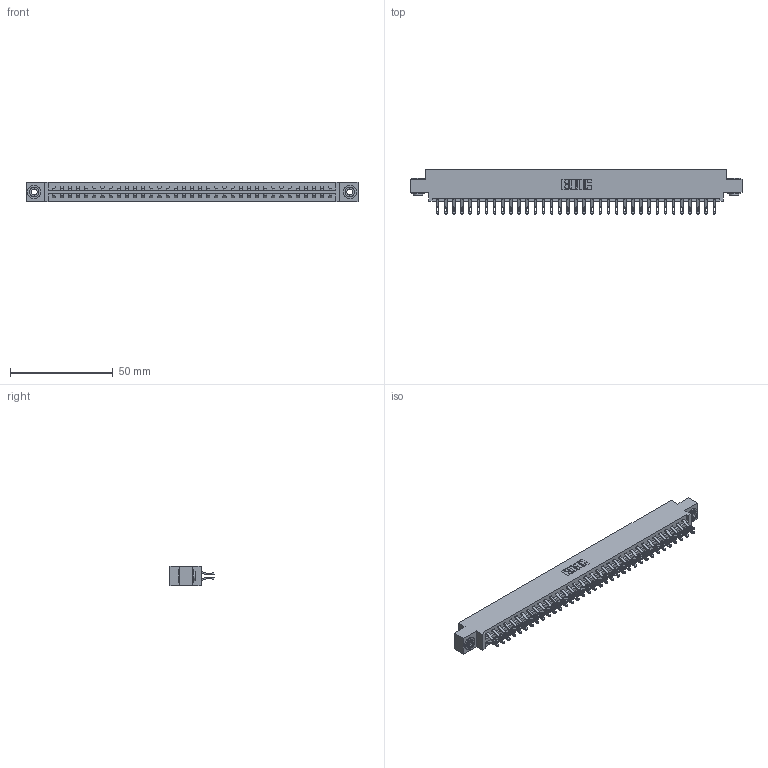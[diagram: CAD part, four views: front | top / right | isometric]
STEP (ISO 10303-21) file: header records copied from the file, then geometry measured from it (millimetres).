
FILE_DESCRIPTION (( 'STEP AP203' ), '1' );
FILE_NAME ('387-070-555-803.STEP', '2018-09-22T17:11:37', ( '' ), ( '' ), 'SwSTEP 2.0', 'SolidWorks 2016', '' );
FILE_SCHEMA (( 'CONFIG_CONTROL_DESIGN' ));
Length unit declared in the file: inch
Products named in the file (4): 337 Part_0.170 Offset - 0.156 Dia-TH; 345-292-001_555 Tail; 345-250-002_345-250-002-102; 387-070-555-803
Assembly tree (73 placements, depth 2):
  387-070-555-803
    337 Part_0.170 Offset - 0.156 Dia-TH
    345-292-001_555 Tail  x70
    345-250-002_345-250-002-102  x2
Bounding box: 161.7 x 21.47 x 9.4 mm (x, y, z)
Volume: 17052.6 mm3; surface area: 20307.4 mm2
Topology: 73 solids, 73 shells, 4356 faces, 13629 edges, 9082 vertices
Faces by surface type: plane 2604, cylinder 1744, cone 8
Entity records: 29150 total; most frequent: CARTESIAN_POINT 4927, ORIENTED_EDGE 4826, DIRECTION 4207, EDGE_CURVE 2413, LINE 2241, VECTOR 2241, VERTEX_POINT 1606, AXIS2_PLACEMENT_3D 983
